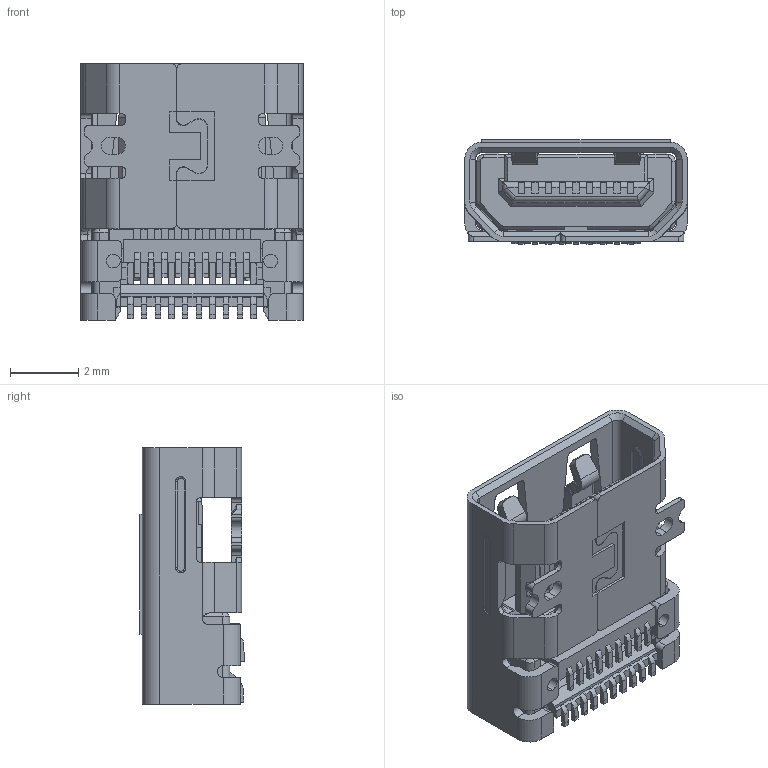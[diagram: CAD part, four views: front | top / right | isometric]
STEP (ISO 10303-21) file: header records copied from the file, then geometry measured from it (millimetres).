
FILE_DESCRIPTION (( 'STEP AP214' ), '1' );
FILE_NAME ('694H319-166-211.STEP', '2021-01-13T18:47:51', ( '' ), ( '' ), 'SwSTEP 2.0', 'SolidWorks 2020', '' );
FILE_SCHEMA (( 'AUTOMOTIVE_DESIGN' ));
Length unit declared in the file: millimetre
Products named in the file (4): 694H319-166-211; Insulator 694H319-X66-211; Tape 694H319-X66-211; Shell 694H319-X66-211
Assembly tree (3 placements, depth 2):
  694H319-166-211
    Insulator 694H319-X66-211
    Shell 694H319-X66-211
    Tape 694H319-X66-211
Bounding box: 6.5 x 3.06 x 7.5 mm (x, y, z)
Volume: 61.8 mm3; surface area: 457.2 mm2
Topology: 3 solids, 3 shells, 1385 faces, 4082 edges, 2621 vertices
Faces by surface type: plane 1104, cylinder 221, cone 37, bspline 21, torus 2
Entity records: 58235 total; most frequent: CARTESIAN_POINT 10961, ORIENTED_EDGE 8164, DIRECTION 6460, EDGE_CURVE 4082, LINE 3178, VECTOR 3178, VERTEX_POINT 2621, AXIS2_PLACEMENT_3D 1641
